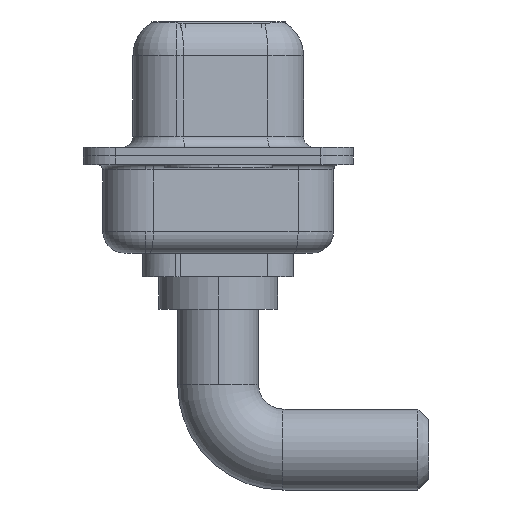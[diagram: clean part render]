
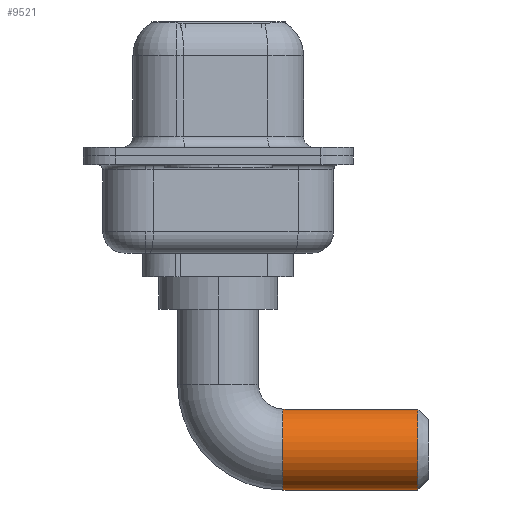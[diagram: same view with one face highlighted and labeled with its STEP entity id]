
A CAD part, left-side view. The second image highlights one B-rep face of the part: STEP entity #9521.
In plain terms, the highlighted cylindrical face has radius 1.875 mm (diameter 3.75 mm), a partial arc.
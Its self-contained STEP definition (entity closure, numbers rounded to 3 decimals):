
#34 = CARTESIAN_POINT ( 'NONE',  ( 0., -3., -6.5 ) ) ;
#40 = AXIS2_PLACEMENT_3D ( 'NONE', #34, #2746, #8793 ) ;
#114 = LINE ( 'NONE', #5207, #1548 ) ;
#181 = VERTEX_POINT ( 'NONE', #9153 ) ;
#403 = CARTESIAN_POINT ( 'NONE',  ( 0., -9.25, -6.5 ) ) ;
#577 = VECTOR ( 'NONE', #1643, 1000. ) ;
#1044 = DIRECTION ( 'NONE',  ( 0., -1., 0. ) ) ;
#1096 = CARTESIAN_POINT ( 'NONE',  ( 0., -3., -4.625 ) ) ;
#1286 = VERTEX_POINT ( 'NONE', #1096 ) ;
#1423 = CARTESIAN_POINT ( 'NONE',  ( 0., -3., -8.375 ) ) ;
#1537 = VERTEX_POINT ( 'NONE', #1423 ) ;
#1548 = VECTOR ( 'NONE', #1044, 1000. ) ;
#1643 = DIRECTION ( 'NONE',  ( 0., -1., 0. ) ) ;
#1878 = EDGE_CURVE ( 'NONE', #1286, #1537, #9887, .T. ) ;
#2161 = DIRECTION ( 'NONE',  ( -1., 0., 0. ) ) ;
#2746 = DIRECTION ( 'NONE',  ( 0., -1., 0. ) ) ;
#2923 = AXIS2_PLACEMENT_3D ( 'NONE', #403, #7701, #10152 ) ;
#3188 = ORIENTED_EDGE ( 'NONE', *, *, #11476, .F. ) ;
#3415 = VERTEX_POINT ( 'NONE', #10579 ) ;
#3672 = CIRCLE ( 'NONE', #2923, 1.875 ) ;
#4430 = CYLINDRICAL_SURFACE ( 'NONE', #40, 1.875 ) ;
#4869 = AXIS2_PLACEMENT_3D ( 'NONE', #8316, #10127, #2161 ) ;
#5207 = CARTESIAN_POINT ( 'NONE',  ( 0., -3., -4.625 ) ) ;
#5490 = EDGE_CURVE ( 'NONE', #181, #3415, #3672, .T. ) ;
#6118 = FACE_OUTER_BOUND ( 'NONE', #7764, .T. ) ;
#6948 = ORIENTED_EDGE ( 'NONE', *, *, #5490, .T. ) ;
#7701 = DIRECTION ( 'NONE',  ( 0., 1., 0. ) ) ;
#7764 = EDGE_LOOP ( 'NONE', ( #3188, #11400, #7889, #6948 ) ) ;
#7889 = ORIENTED_EDGE ( 'NONE', *, *, #9430, .T. ) ;
#7963 = LINE ( 'NONE', #8969, #577 ) ;
#8316 = CARTESIAN_POINT ( 'NONE',  ( 0., -3., -6.5 ) ) ;
#8793 = DIRECTION ( 'NONE',  ( 0., 0., -1. ) ) ;
#8969 = CARTESIAN_POINT ( 'NONE',  ( 0., -3., -8.375 ) ) ;
#9153 = CARTESIAN_POINT ( 'NONE',  ( 0., -9.25, -8.375 ) ) ;
#9430 = EDGE_CURVE ( 'NONE', #1537, #181, #7963, .T. ) ;
#9521 = ADVANCED_FACE ( 'NONE', ( #6118 ), #4430, .T. ) ;
#9887 = CIRCLE ( 'NONE', #4869, 1.875 ) ;
#10127 = DIRECTION ( 'NONE',  ( 0., -1., 0. ) ) ;
#10152 = DIRECTION ( 'NONE',  ( 0., 0., -1. ) ) ;
#10579 = CARTESIAN_POINT ( 'NONE',  ( 0., -9.25, -4.625 ) ) ;
#11400 = ORIENTED_EDGE ( 'NONE', *, *, #1878, .T. ) ;
#11476 = EDGE_CURVE ( 'NONE', #1286, #3415, #114, .T. ) ;
